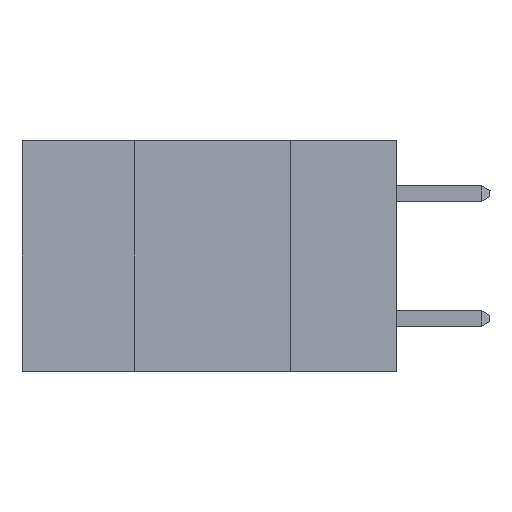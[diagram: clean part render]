
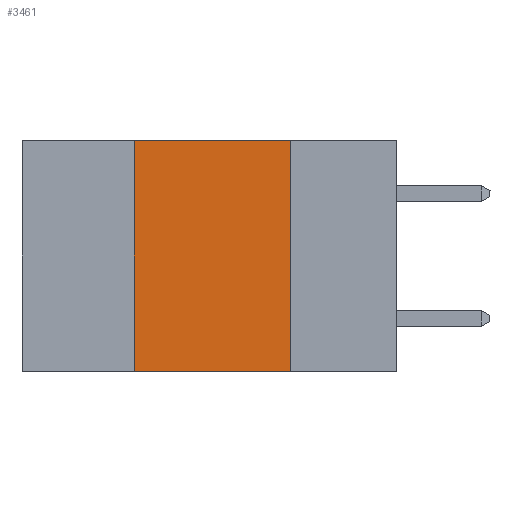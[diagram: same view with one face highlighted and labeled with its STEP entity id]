
A CAD part, left-side view. The second image highlights one B-rep face of the part: STEP entity #3461.
In plain terms, the highlighted planar face has unit normal (-1, 0, 0).
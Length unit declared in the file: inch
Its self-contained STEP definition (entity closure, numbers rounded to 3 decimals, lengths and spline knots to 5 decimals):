
#610 = DIRECTION ( 'NONE',  ( 0., 0., 1. ) ) ;
#693 = EDGE_CURVE ( 'NONE', #4662, #12252, #11192, .T. ) ;
#1380 = CARTESIAN_POINT ( 'NONE',  ( 0., 0.42, 0. ) ) ;
#1387 = VERTEX_POINT ( 'NONE', #2574 ) ;
#1474 = CARTESIAN_POINT ( 'NONE',  ( 0., 0.17, 0. ) ) ;
#1976 = LINE ( 'NONE', #12775, #12288 ) ;
#2574 = CARTESIAN_POINT ( 'NONE',  ( 0., 0.42, 0. ) ) ;
#3329 = CARTESIAN_POINT ( 'NONE',  ( 0., 0.6, -0.37 ) ) ;
#3461 = ADVANCED_FACE ( 'NONE', ( #7658 ), #3966, .F. ) ;
#3486 = DIRECTION ( 'NONE',  ( 0., -1., 0. ) ) ;
#3841 = CARTESIAN_POINT ( 'NONE',  ( 0., 0.42, -0.37 ) ) ;
#3966 = PLANE ( 'NONE',  #4862 ) ;
#4475 = ORIENTED_EDGE ( 'NONE', *, *, #11672, .F. ) ;
#4647 = DIRECTION ( 'NONE',  ( 0., -1., 0. ) ) ;
#4662 = VERTEX_POINT ( 'NONE', #3841 ) ;
#4862 = AXIS2_PLACEMENT_3D ( 'NONE', #7858, #7913, #11375 ) ;
#5099 = EDGE_CURVE ( 'NONE', #1387, #5949, #8910, .T. ) ;
#5462 = ORIENTED_EDGE ( 'NONE', *, *, #5099, .F. ) ;
#5484 = EDGE_LOOP ( 'NONE', ( #4475, #5462, #10617, #10325 ) ) ;
#5767 = DIRECTION ( 'NONE',  ( 0., 0., -1. ) ) ;
#5810 = EDGE_CURVE ( 'NONE', #4662, #1387, #11084, .T. ) ;
#5942 = VECTOR ( 'NONE', #610, 39.37008 ) ;
#5949 = VERTEX_POINT ( 'NONE', #1474 ) ;
#6959 = CARTESIAN_POINT ( 'NONE',  ( 0., 0.6, 0. ) ) ;
#7557 = CARTESIAN_POINT ( 'NONE',  ( 0., 0.17, -0.37 ) ) ;
#7658 = FACE_OUTER_BOUND ( 'NONE', #5484, .T. ) ;
#7858 = CARTESIAN_POINT ( 'NONE',  ( 0., 0.6, 0. ) ) ;
#7913 = DIRECTION ( 'NONE',  ( 1., 0., 0. ) ) ;
#8261 = VECTOR ( 'NONE', #4647, 39.37008 ) ;
#8523 = VECTOR ( 'NONE', #3486, 39.37008 ) ;
#8910 = LINE ( 'NONE', #6959, #8261 ) ;
#10325 = ORIENTED_EDGE ( 'NONE', *, *, #693, .T. ) ;
#10617 = ORIENTED_EDGE ( 'NONE', *, *, #5810, .F. ) ;
#11084 = LINE ( 'NONE', #1380, #5942 ) ;
#11192 = LINE ( 'NONE', #3329, #8523 ) ;
#11375 = DIRECTION ( 'NONE',  ( 0., 0., -1. ) ) ;
#11672 = EDGE_CURVE ( 'NONE', #5949, #12252, #1976, .T. ) ;
#12252 = VERTEX_POINT ( 'NONE', #7557 ) ;
#12288 = VECTOR ( 'NONE', #5767, 39.37008 ) ;
#12775 = CARTESIAN_POINT ( 'NONE',  ( 0., 0.17, 0. ) ) ;
